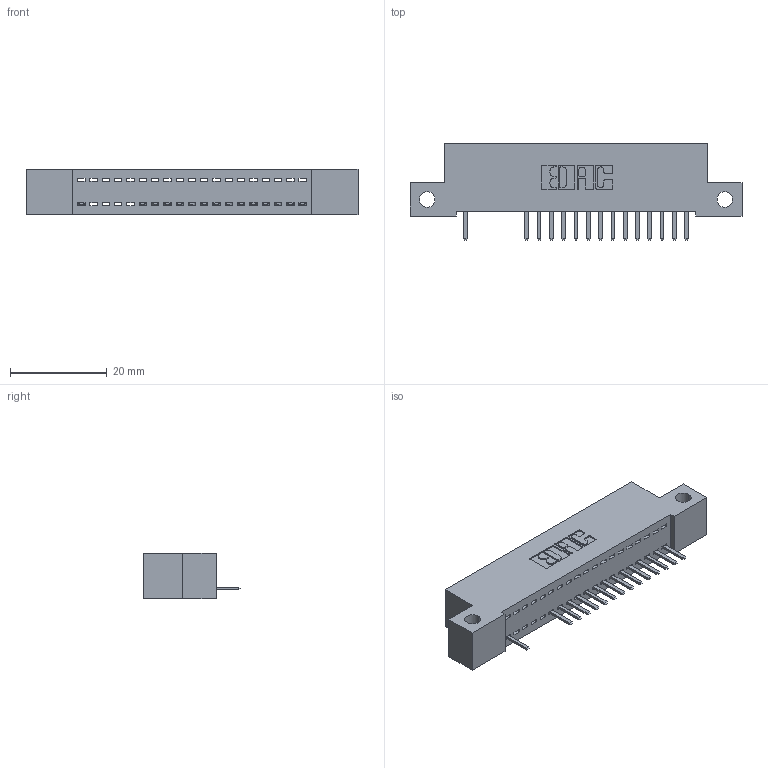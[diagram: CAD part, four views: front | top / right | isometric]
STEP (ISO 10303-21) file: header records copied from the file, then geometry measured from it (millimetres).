
FILE_DESCRIPTION (( 'STEP AP203' ), '1' );
FILE_NAME ('392-019-520-112.STEP', '2018-08-15T05:09:09', ( '' ), ( '' ), 'SwSTEP 2.0', 'SolidWorks 2016', '' );
FILE_SCHEMA (( 'CONFIG_CONTROL_DESIGN' ));
Length unit declared in the file: inch
Products named in the file (3): 342 Part_Side Mount; 345-292-001_345-293-120; 392-019-520-112
Assembly tree (16 placements, depth 2):
  392-019-520-112
    342 Part_Side Mount
    345-292-001_345-293-120  x15
Bounding box: 68.58 x 20.02 x 9.4 mm (x, y, z)
Volume: 5765.6 mm3; surface area: 7498.9 mm2
Topology: 16 solids, 16 shells, 1088 faces, 3227 edges, 2110 vertices
Faces by surface type: plane 774, cylinder 314
Entity records: 14447 total; most frequent: CARTESIAN_POINT 2531, ORIENTED_EDGE 2478, DIRECTION 2165, EDGE_CURVE 1239, LINE 1107, VECTOR 1107, VERTEX_POINT 822, AXIS2_PLACEMENT_3D 529
